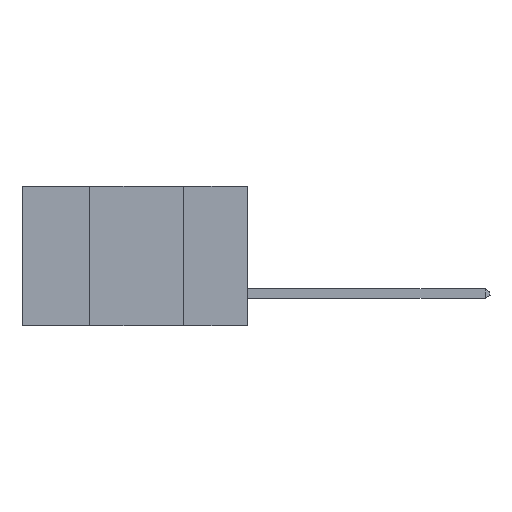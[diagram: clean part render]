
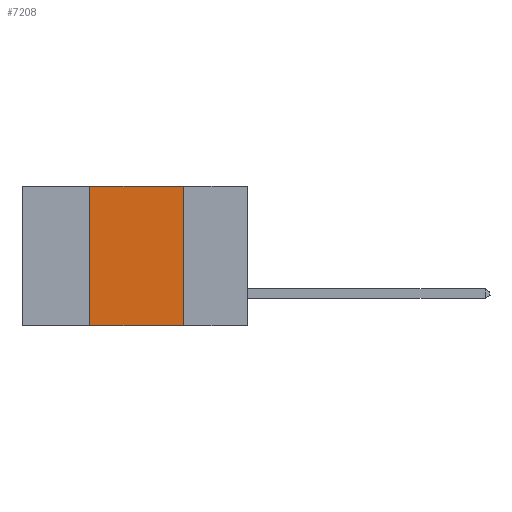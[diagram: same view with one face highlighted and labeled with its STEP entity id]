
A CAD part, left-side view. The second image highlights one B-rep face of the part: STEP entity #7208.
In plain terms, the highlighted planar face has unit normal (-1, 0, 0).
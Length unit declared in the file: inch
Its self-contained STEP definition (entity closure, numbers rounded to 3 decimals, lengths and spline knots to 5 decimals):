
#80 = VERTEX_POINT ( 'NONE', #10965 ) ;
#495 = CARTESIAN_POINT ( 'NONE',  ( 0., 0.17, -0.37 ) ) ;
#538 = LINE ( 'NONE', #1153, #3823 ) ;
#644 = EDGE_LOOP ( 'NONE', ( #11414, #6553, #12273, #5352 ) ) ;
#1141 = DIRECTION ( 'NONE',  ( 0., 0., -1. ) ) ;
#1153 = CARTESIAN_POINT ( 'NONE',  ( 0., 0.6, -0.37 ) ) ;
#1490 = AXIS2_PLACEMENT_3D ( 'NONE', #4131, #10782, #1141 ) ;
#1925 = VECTOR ( 'NONE', #5152, 39.37008 ) ;
#2384 = VECTOR ( 'NONE', #5616, 39.37008 ) ;
#2758 = CARTESIAN_POINT ( 'NONE',  ( 0., 0.6, 0. ) ) ;
#2896 = DIRECTION ( 'NONE',  ( 0., -1., 0. ) ) ;
#3703 = VECTOR ( 'NONE', #6429, 39.37008 ) ;
#3823 = VECTOR ( 'NONE', #2896, 39.37008 ) ;
#4131 = CARTESIAN_POINT ( 'NONE',  ( 0., 0.6, 0. ) ) ;
#4556 = VERTEX_POINT ( 'NONE', #495 ) ;
#4860 = FACE_OUTER_BOUND ( 'NONE', #644, .T. ) ;
#5152 = DIRECTION ( 'NONE',  ( 0., 0., -1. ) ) ;
#5352 = ORIENTED_EDGE ( 'NONE', *, *, #7659, .T. ) ;
#5488 = VERTEX_POINT ( 'NONE', #11898 ) ;
#5531 = EDGE_CURVE ( 'NONE', #6156, #4556, #5940, .T. ) ;
#5616 = DIRECTION ( 'NONE',  ( 0., 0., 1. ) ) ;
#5913 = PLANE ( 'NONE',  #1490 ) ;
#5940 = LINE ( 'NONE', #8005, #1925 ) ;
#6156 = VERTEX_POINT ( 'NONE', #11662 ) ;
#6227 = LINE ( 'NONE', #2758, #3703 ) ;
#6429 = DIRECTION ( 'NONE',  ( 0., -1., 0. ) ) ;
#6553 = ORIENTED_EDGE ( 'NONE', *, *, #6910, .F. ) ;
#6910 = EDGE_CURVE ( 'NONE', #80, #6156, #6227, .T. ) ;
#7208 = ADVANCED_FACE ( 'NONE', ( #4860 ), #5913, .F. ) ;
#7316 = LINE ( 'NONE', #12200, #2384 ) ;
#7659 = EDGE_CURVE ( 'NONE', #5488, #4556, #538, .T. ) ;
#8005 = CARTESIAN_POINT ( 'NONE',  ( 0., 0.17, 0. ) ) ;
#10410 = EDGE_CURVE ( 'NONE', #5488, #80, #7316, .T. ) ;
#10782 = DIRECTION ( 'NONE',  ( 1., 0., 0. ) ) ;
#10965 = CARTESIAN_POINT ( 'NONE',  ( 0., 0.42, 0. ) ) ;
#11414 = ORIENTED_EDGE ( 'NONE', *, *, #5531, .F. ) ;
#11662 = CARTESIAN_POINT ( 'NONE',  ( 0., 0.17, 0. ) ) ;
#11898 = CARTESIAN_POINT ( 'NONE',  ( 0., 0.42, -0.37 ) ) ;
#12200 = CARTESIAN_POINT ( 'NONE',  ( 0., 0.42, 0. ) ) ;
#12273 = ORIENTED_EDGE ( 'NONE', *, *, #10410, .F. ) ;
